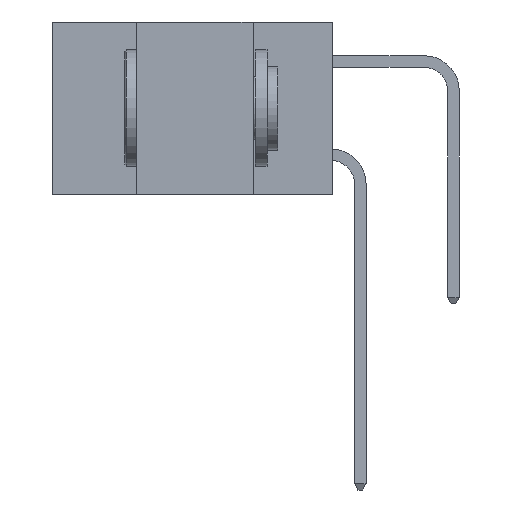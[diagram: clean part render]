
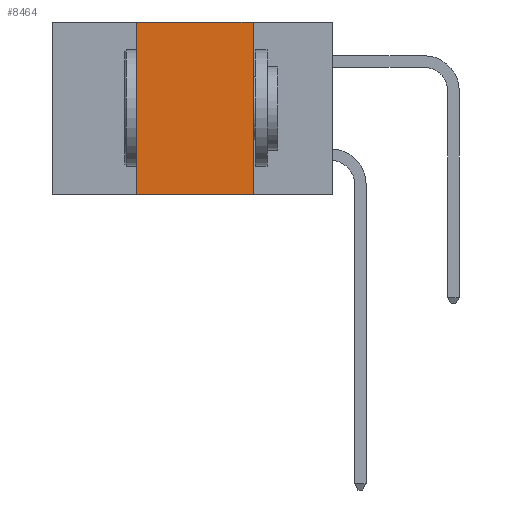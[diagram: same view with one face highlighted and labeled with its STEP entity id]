
A CAD part, left-side view. The second image highlights one B-rep face of the part: STEP entity #8464.
In plain terms, the highlighted planar face has unit normal (-1, 0, 0).
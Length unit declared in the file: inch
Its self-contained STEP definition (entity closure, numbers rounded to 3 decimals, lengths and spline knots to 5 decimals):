
#568 = DIRECTION ( 'NONE',  ( 0., 0., -1. ) ) ;
#2375 = CARTESIAN_POINT ( 'NONE',  ( 0., 0.17, 0. ) ) ;
#2652 = VERTEX_POINT ( 'NONE', #2375 ) ;
#3388 = PLANE ( 'NONE',  #3892 ) ;
#3636 = EDGE_LOOP ( 'NONE', ( #18369, #24582, #22338, #23650 ) ) ;
#3892 = AXIS2_PLACEMENT_3D ( 'NONE', #22279, #9659, #24356 ) ;
#4441 = VERTEX_POINT ( 'NONE', #16861 ) ;
#6337 = CARTESIAN_POINT ( 'NONE',  ( 0., 0.42, -0.37 ) ) ;
#7123 = DIRECTION ( 'NONE',  ( 0., -1., 0. ) ) ;
#8464 = ADVANCED_FACE ( 'NONE', ( #8740 ), #3388, .F. ) ;
#8740 = FACE_OUTER_BOUND ( 'NONE', #3636, .T. ) ;
#8916 = EDGE_CURVE ( 'NONE', #2652, #4441, #26114, .T. ) ;
#9659 = DIRECTION ( 'NONE',  ( 1., 0., 0. ) ) ;
#10709 = VERTEX_POINT ( 'NONE', #20688 ) ;
#11223 = CARTESIAN_POINT ( 'NONE',  ( 0., 0.6, 0. ) ) ;
#12272 = LINE ( 'NONE', #6337, #22796 ) ;
#12583 = VERTEX_POINT ( 'NONE', #25159 ) ;
#13592 = VECTOR ( 'NONE', #15541, 39.37008 ) ;
#14691 = DIRECTION ( 'NONE',  ( 0., 0., 1. ) ) ;
#15179 = CARTESIAN_POINT ( 'NONE',  ( 0., 0.17, -0.37 ) ) ;
#15541 = DIRECTION ( 'NONE',  ( 0., -1., 0. ) ) ;
#15636 = EDGE_CURVE ( 'NONE', #12583, #2652, #19163, .T. ) ;
#16848 = EDGE_CURVE ( 'NONE', #10709, #4441, #23696, .T. ) ;
#16861 = CARTESIAN_POINT ( 'NONE',  ( 0., 0.17, -0.37 ) ) ;
#18369 = ORIENTED_EDGE ( 'NONE', *, *, #8916, .F. ) ;
#19163 = LINE ( 'NONE', #11223, #13592 ) ;
#19681 = CARTESIAN_POINT ( 'NONE',  ( 0., 0.6, -0.37 ) ) ;
#20688 = CARTESIAN_POINT ( 'NONE',  ( 0., 0.42, -0.37 ) ) ;
#22279 = CARTESIAN_POINT ( 'NONE',  ( 0., 0.6, 0. ) ) ;
#22338 = ORIENTED_EDGE ( 'NONE', *, *, #24217, .F. ) ;
#22796 = VECTOR ( 'NONE', #14691, 39.37008 ) ;
#23037 = VECTOR ( 'NONE', #7123, 39.37008 ) ;
#23650 = ORIENTED_EDGE ( 'NONE', *, *, #16848, .T. ) ;
#23696 = LINE ( 'NONE', #19681, #23037 ) ;
#24217 = EDGE_CURVE ( 'NONE', #10709, #12583, #12272, .T. ) ;
#24356 = DIRECTION ( 'NONE',  ( 0., 0., -1. ) ) ;
#24582 = ORIENTED_EDGE ( 'NONE', *, *, #15636, .F. ) ;
#25159 = CARTESIAN_POINT ( 'NONE',  ( 0., 0.42, 0. ) ) ;
#26114 = LINE ( 'NONE', #15179, #26761 ) ;
#26761 = VECTOR ( 'NONE', #568, 39.37008 ) ;
